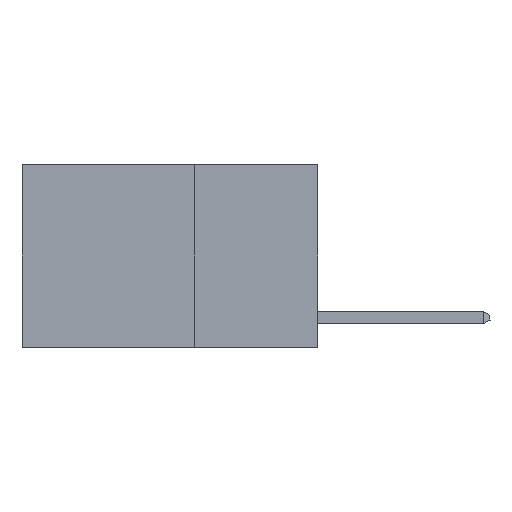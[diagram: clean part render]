
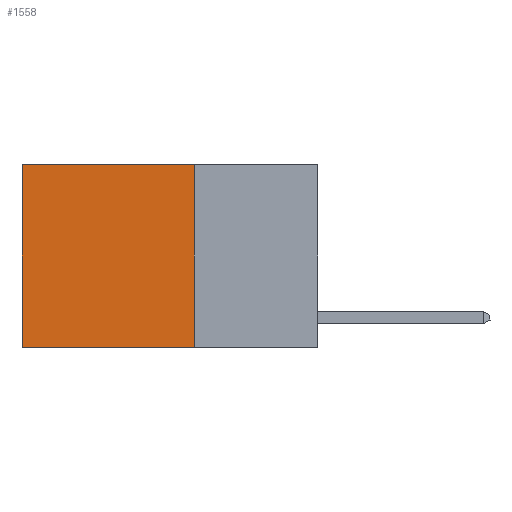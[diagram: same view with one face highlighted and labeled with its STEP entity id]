
A CAD part, left-side view. The second image highlights one B-rep face of the part: STEP entity #1558.
In plain terms, the highlighted planar face has unit normal (-1, 0, 0).
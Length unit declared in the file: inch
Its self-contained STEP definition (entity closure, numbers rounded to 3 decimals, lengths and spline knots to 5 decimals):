
#98 = CARTESIAN_POINT ( 'NONE',  ( 0.2625, 0.6, 0. ) ) ;
#289 = EDGE_CURVE ( 'NONE', #4034, #8136, #2192, .T. ) ;
#359 = ORIENTED_EDGE ( 'NONE', *, *, #289, .T. ) ;
#598 = CARTESIAN_POINT ( 'NONE',  ( 0.2625, 0.6, -0.37 ) ) ;
#612 = DIRECTION ( 'NONE',  ( 0., 0., -1. ) ) ;
#771 = EDGE_CURVE ( 'NONE', #8136, #2489, #6362, .T. ) ;
#1242 = LINE ( 'NONE', #8582, #8008 ) ;
#1558 = ADVANCED_FACE ( 'NONE', ( #3211 ), #4228, .F. ) ;
#1649 = EDGE_LOOP ( 'NONE', ( #7779, #5395, #1760, #359 ) ) ;
#1760 = ORIENTED_EDGE ( 'NONE', *, *, #7213, .F. ) ;
#1813 = CARTESIAN_POINT ( 'NONE',  ( 0.2625, 0.25, -0.37 ) ) ;
#2158 = DIRECTION ( 'NONE',  ( 0., 0., -1. ) ) ;
#2192 = LINE ( 'NONE', #6417, #3735 ) ;
#2249 = CARTESIAN_POINT ( 'NONE',  ( 0.2625, 0.25, 0. ) ) ;
#2489 = VERTEX_POINT ( 'NONE', #598 ) ;
#2937 = VECTOR ( 'NONE', #612, 39.37008 ) ;
#3211 = FACE_OUTER_BOUND ( 'NONE', #1649, .T. ) ;
#3650 = DIRECTION ( 'NONE',  ( 0., 1., 0. ) ) ;
#3735 = VECTOR ( 'NONE', #3650, 39.37008 ) ;
#3970 = DIRECTION ( 'NONE',  ( 0., 0., -1. ) ) ;
#4020 = DIRECTION ( 'NONE',  ( 1., 0., 0. ) ) ;
#4034 = VERTEX_POINT ( 'NONE', #2249 ) ;
#4036 = EDGE_CURVE ( 'NONE', #5120, #2489, #6608, .T. ) ;
#4228 = PLANE ( 'NONE',  #8607 ) ;
#4397 = CARTESIAN_POINT ( 'NONE',  ( 0.2625, 0.25, 0. ) ) ;
#4893 = VECTOR ( 'NONE', #6789, 39.37008 ) ;
#5120 = VERTEX_POINT ( 'NONE', #1813 ) ;
#5395 = ORIENTED_EDGE ( 'NONE', *, *, #4036, .F. ) ;
#5507 = CARTESIAN_POINT ( 'NONE',  ( 0.2625, 0.25, -0.37 ) ) ;
#6362 = LINE ( 'NONE', #7375, #2937 ) ;
#6417 = CARTESIAN_POINT ( 'NONE',  ( 0.2625, 0.25, 0. ) ) ;
#6608 = LINE ( 'NONE', #5507, #4893 ) ;
#6789 = DIRECTION ( 'NONE',  ( 0., 1., 0. ) ) ;
#7213 = EDGE_CURVE ( 'NONE', #4034, #5120, #1242, .T. ) ;
#7375 = CARTESIAN_POINT ( 'NONE',  ( 0.2625, 0.6, 0. ) ) ;
#7779 = ORIENTED_EDGE ( 'NONE', *, *, #771, .T. ) ;
#8008 = VECTOR ( 'NONE', #2158, 39.37008 ) ;
#8136 = VERTEX_POINT ( 'NONE', #98 ) ;
#8582 = CARTESIAN_POINT ( 'NONE',  ( 0.2625, 0.25, 0. ) ) ;
#8607 = AXIS2_PLACEMENT_3D ( 'NONE', #4397, #4020, #3970 ) ;
